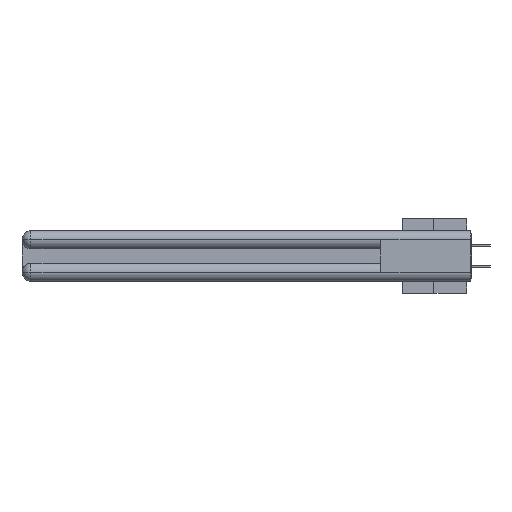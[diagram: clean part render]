
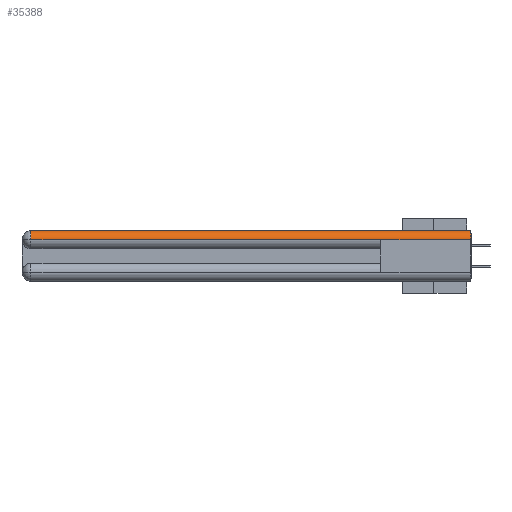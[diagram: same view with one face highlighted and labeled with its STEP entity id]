
A CAD part, left-side view. The second image highlights one B-rep face of the part: STEP entity #35388.
In plain terms, the highlighted cylindrical face has radius 1.562 mm (diameter 3.124 mm), a partial arc.
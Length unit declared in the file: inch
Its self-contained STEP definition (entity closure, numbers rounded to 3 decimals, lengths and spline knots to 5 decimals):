
#1605 = CARTESIAN_POINT ( 'NONE',  ( 0.0615, 0., -0.0615 ) ) ;
#2292 = CIRCLE ( 'NONE', #15069, 0.0615 ) ;
#4028 = VERTEX_POINT ( 'NONE', #18583 ) ;
#4219 = CIRCLE ( 'NONE', #28800, 0.0615 ) ;
#5373 = EDGE_CURVE ( 'NONE', #32100, #28435, #11336, .T. ) ;
#7159 = AXIS2_PLACEMENT_3D ( 'NONE', #33758, #33610, #27490 ) ;
#8439 = LINE ( 'NONE', #22504, #24788 ) ;
#8736 = ORIENTED_EDGE ( 'NONE', *, *, #15511, .T. ) ;
#9630 = ORIENTED_EDGE ( 'NONE', *, *, #18364, .F. ) ;
#10953 = DIRECTION ( 'NONE',  ( 0., 0., 1. ) ) ;
#11146 = DIRECTION ( 'NONE',  ( 1., 0., 0. ) ) ;
#11336 = LINE ( 'NONE', #16947, #23632 ) ;
#12467 = ORIENTED_EDGE ( 'NONE', *, *, #33625, .T. ) ;
#14565 = DIRECTION ( 'NONE',  ( 0., -1., 0. ) ) ;
#15069 = AXIS2_PLACEMENT_3D ( 'NONE', #33752, #40295, #10953 ) ;
#15511 = EDGE_CURVE ( 'NONE', #21295, #32649, #2292, .T. ) ;
#16947 = CARTESIAN_POINT ( 'NONE',  ( 0., 3., -0.0615 ) ) ;
#18043 = ORIENTED_EDGE ( 'NONE', *, *, #29796, .F. ) ;
#18364 = EDGE_CURVE ( 'NONE', #21295, #4028, #35682, .T. ) ;
#18583 = CARTESIAN_POINT ( 'NONE',  ( 0.0615, 0., 0. ) ) ;
#19509 = CARTESIAN_POINT ( 'NONE',  ( 0., 0., -0.0615 ) ) ;
#21295 = VERTEX_POINT ( 'NONE', #38125 ) ;
#21562 = FACE_OUTER_BOUND ( 'NONE', #34291, .T. ) ;
#22504 = CARTESIAN_POINT ( 'NONE',  ( 0., 3., -0.0615 ) ) ;
#23632 = VECTOR ( 'NONE', #26775, 39.37008 ) ;
#24788 = VECTOR ( 'NONE', #41724, 39.37008 ) ;
#26422 = CARTESIAN_POINT ( 'NONE',  ( 0.0615, 0., 0. ) ) ;
#26775 = DIRECTION ( 'NONE',  ( 0., 1., 0. ) ) ;
#27490 = DIRECTION ( 'NONE',  ( 0., 0., 1. ) ) ;
#28435 = VERTEX_POINT ( 'NONE', #28923 ) ;
#28800 = AXIS2_PLACEMENT_3D ( 'NONE', #1605, #14565, #11146 ) ;
#28923 = CARTESIAN_POINT ( 'NONE',  ( 0., 0.6, -0.0615 ) ) ;
#29176 = CYLINDRICAL_SURFACE ( 'NONE', #7159, 0.0615 ) ;
#29484 = ORIENTED_EDGE ( 'NONE', *, *, #5373, .F. ) ;
#29796 = EDGE_CURVE ( 'NONE', #4028, #32100, #4219, .T. ) ;
#32100 = VERTEX_POINT ( 'NONE', #19509 ) ;
#32649 = VERTEX_POINT ( 'NONE', #32971 ) ;
#32971 = CARTESIAN_POINT ( 'NONE',  ( 0., 2.94, -0.0615 ) ) ;
#33610 = DIRECTION ( 'NONE',  ( 0., 1., 0. ) ) ;
#33625 = EDGE_CURVE ( 'NONE', #32649, #28435, #8439, .T. ) ;
#33752 = CARTESIAN_POINT ( 'NONE',  ( 0.0615, 2.94, -0.0615 ) ) ;
#33758 = CARTESIAN_POINT ( 'NONE',  ( 0.0615, 0., -0.0615 ) ) ;
#34291 = EDGE_LOOP ( 'NONE', ( #9630, #8736, #12467, #29484, #18043 ) ) ;
#35388 = ADVANCED_FACE ( 'NONE', ( #21562 ), #29176, .T. ) ;
#35682 = LINE ( 'NONE', #26422, #37219 ) ;
#37219 = VECTOR ( 'NONE', #42222, 39.37008 ) ;
#38125 = CARTESIAN_POINT ( 'NONE',  ( 0.0615, 2.94, 0. ) ) ;
#40295 = DIRECTION ( 'NONE',  ( 0., -1., 0. ) ) ;
#41724 = DIRECTION ( 'NONE',  ( 0., -1., 0. ) ) ;
#42222 = DIRECTION ( 'NONE',  ( 0., -1., 0. ) ) ;
